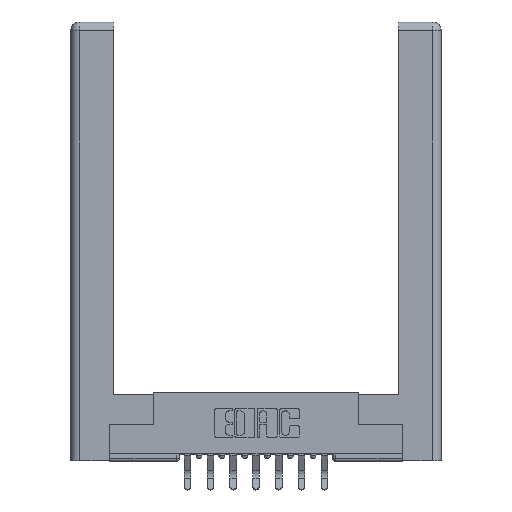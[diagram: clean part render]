
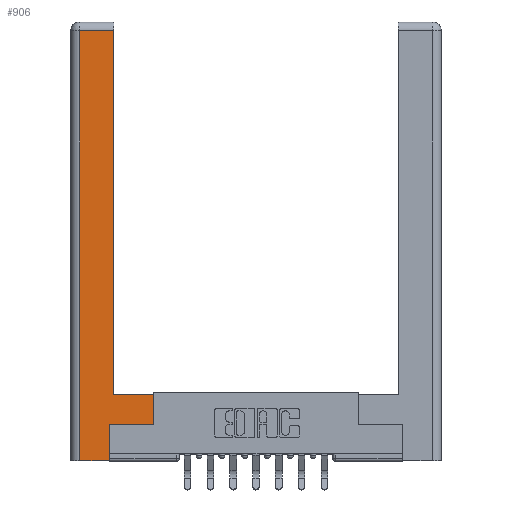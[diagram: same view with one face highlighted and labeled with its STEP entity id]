
A CAD part, top view. The second image highlights one B-rep face of the part: STEP entity #906.
In plain terms, the highlighted planar face has unit normal (0, 0, 1).
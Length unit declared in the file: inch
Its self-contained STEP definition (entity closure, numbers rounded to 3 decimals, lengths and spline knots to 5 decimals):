
#92 = CARTESIAN_POINT ( 'NONE',  ( 0.295, 2.94, 0. ) ) ;
#177 = CARTESIAN_POINT ( 'NONE',  ( 0.295, 0.45, 0. ) ) ;
#330 = CARTESIAN_POINT ( 'NONE',  ( 0.0615, 2.94, 0. ) ) ;
#458 = LINE ( 'NONE', #330, #2925 ) ;
#883 = CARTESIAN_POINT ( 'NONE',  ( 0.565, 0.245, 0. ) ) ;
#899 = VECTOR ( 'NONE', #10425, 39.37008 ) ;
#906 = ADVANCED_FACE ( 'NONE', ( #6199 ), #10125, .F. ) ;
#907 = DIRECTION ( 'NONE',  ( 0., 1., 0. ) ) ;
#980 = AXIS2_PLACEMENT_3D ( 'NONE', #12286, #10323, #6938 ) ;
#1039 = ORIENTED_EDGE ( 'NONE', *, *, #10851, .T. ) ;
#1232 = CARTESIAN_POINT ( 'NONE',  ( 0.265, 0.245, 0. ) ) ;
#1908 = ORIENTED_EDGE ( 'NONE', *, *, #7429, .T. ) ;
#2039 = VECTOR ( 'NONE', #11423, 39.37008 ) ;
#2101 = CARTESIAN_POINT ( 'NONE',  ( 0.565, 0.245, 0. ) ) ;
#2911 = CARTESIAN_POINT ( 'NONE',  ( 0.565, 0.45, 0. ) ) ;
#2925 = VECTOR ( 'NONE', #12792, 39.37008 ) ;
#3074 = ORIENTED_EDGE ( 'NONE', *, *, #5281, .T. ) ;
#3113 = LINE ( 'NONE', #2101, #6047 ) ;
#3175 = DIRECTION ( 'NONE',  ( 1., 0., 0. ) ) ;
#3181 = CARTESIAN_POINT ( 'NONE',  ( 0.0615, 2.94, 0. ) ) ;
#3234 = ORIENTED_EDGE ( 'NONE', *, *, #10986, .T. ) ;
#3357 = VECTOR ( 'NONE', #3175, 39.37008 ) ;
#3541 = ORIENTED_EDGE ( 'NONE', *, *, #8562, .T. ) ;
#3565 = CARTESIAN_POINT ( 'NONE',  ( 0.0615, 0., 0. ) ) ;
#3612 = EDGE_CURVE ( 'NONE', #4402, #5096, #12589, .T. ) ;
#4402 = VERTEX_POINT ( 'NONE', #3181 ) ;
#5096 = VERTEX_POINT ( 'NONE', #3565 ) ;
#5134 = VERTEX_POINT ( 'NONE', #10691 ) ;
#5160 = CARTESIAN_POINT ( 'NONE',  ( 0.295, 3., 0. ) ) ;
#5281 = EDGE_CURVE ( 'NONE', #12796, #10321, #9259, .T. ) ;
#5288 = VERTEX_POINT ( 'NONE', #7103 ) ;
#5932 = LINE ( 'NONE', #2911, #8633 ) ;
#6047 = VECTOR ( 'NONE', #11405, 39.37008 ) ;
#6052 = LINE ( 'NONE', #11457, #3357 ) ;
#6199 = FACE_OUTER_BOUND ( 'NONE', #10960, .T. ) ;
#6938 = DIRECTION ( 'NONE',  ( -1., 0., 0. ) ) ;
#7103 = CARTESIAN_POINT ( 'NONE',  ( 0.265, 0., 0. ) ) ;
#7276 = CARTESIAN_POINT ( 'NONE',  ( 0.295, 0.45, 0. ) ) ;
#7429 = EDGE_CURVE ( 'NONE', #8832, #5134, #5932, .T. ) ;
#7614 = EDGE_CURVE ( 'NONE', #10430, #8832, #3113, .T. ) ;
#7776 = ORIENTED_EDGE ( 'NONE', *, *, #3612, .T. ) ;
#7930 = VECTOR ( 'NONE', #907, 39.37008 ) ;
#8167 = LINE ( 'NONE', #1232, #2039 ) ;
#8266 = VECTOR ( 'NONE', #11540, 39.37008 ) ;
#8298 = ORIENTED_EDGE ( 'NONE', *, *, #7614, .T. ) ;
#8562 = EDGE_CURVE ( 'NONE', #5288, #10430, #8167, .T. ) ;
#8633 = VECTOR ( 'NONE', #12010, 39.37008 ) ;
#8832 = VERTEX_POINT ( 'NONE', #883 ) ;
#9259 = LINE ( 'NONE', #5160, #7930 ) ;
#10125 = PLANE ( 'NONE',  #980 ) ;
#10306 = EDGE_CURVE ( 'NONE', #5134, #12796, #10386, .T. ) ;
#10321 = VERTEX_POINT ( 'NONE', #92 ) ;
#10323 = DIRECTION ( 'NONE',  ( 0., 0., -1. ) ) ;
#10386 = LINE ( 'NONE', #7276, #8266 ) ;
#10425 = DIRECTION ( 'NONE',  ( 0., -1., 0. ) ) ;
#10430 = VERTEX_POINT ( 'NONE', #13288 ) ;
#10558 = CARTESIAN_POINT ( 'NONE',  ( 0.0615, 0., 0. ) ) ;
#10691 = CARTESIAN_POINT ( 'NONE',  ( 0.565, 0.45, 0. ) ) ;
#10851 = EDGE_CURVE ( 'NONE', #5096, #5288, #6052, .T. ) ;
#10901 = ORIENTED_EDGE ( 'NONE', *, *, #10306, .T. ) ;
#10960 = EDGE_LOOP ( 'NONE', ( #3074, #3234, #7776, #1039, #3541, #8298, #1908, #10901 ) ) ;
#10986 = EDGE_CURVE ( 'NONE', #10321, #4402, #458, .T. ) ;
#11405 = DIRECTION ( 'NONE',  ( 1., 0., 0. ) ) ;
#11423 = DIRECTION ( 'NONE',  ( 0., 1., 0. ) ) ;
#11457 = CARTESIAN_POINT ( 'NONE',  ( 0.265, 0., 0. ) ) ;
#11540 = DIRECTION ( 'NONE',  ( -1., 0., 0. ) ) ;
#12010 = DIRECTION ( 'NONE',  ( 0., 1., 0. ) ) ;
#12286 = CARTESIAN_POINT ( 'NONE',  ( 0., 0., 0. ) ) ;
#12589 = LINE ( 'NONE', #10558, #899 ) ;
#12792 = DIRECTION ( 'NONE',  ( -1., 0., 0. ) ) ;
#12796 = VERTEX_POINT ( 'NONE', #177 ) ;
#13288 = CARTESIAN_POINT ( 'NONE',  ( 0.265, 0.245, 0. ) ) ;
